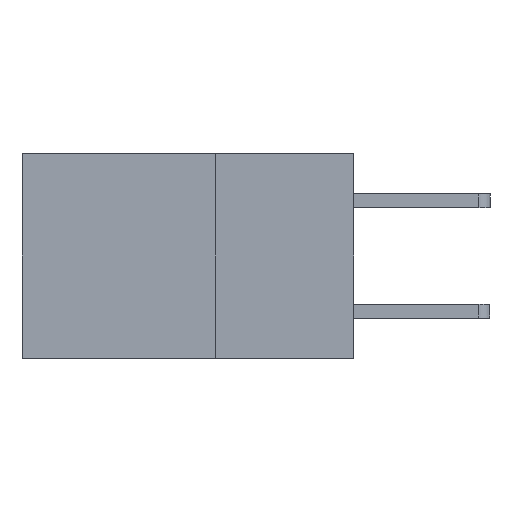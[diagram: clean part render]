
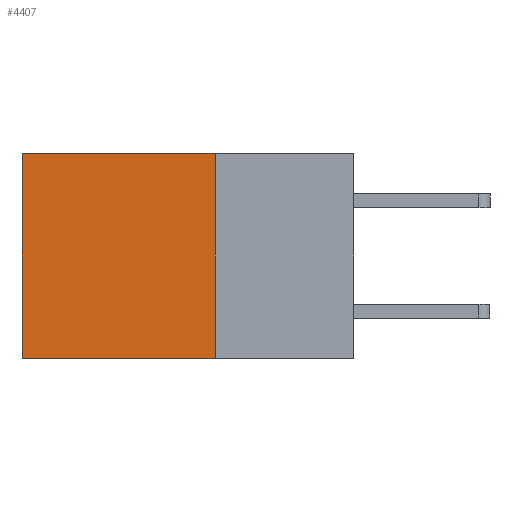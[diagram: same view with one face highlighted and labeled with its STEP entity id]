
A CAD part, left-side view. The second image highlights one B-rep face of the part: STEP entity #4407.
In plain terms, the highlighted planar face has unit normal (-1, 0, 0).
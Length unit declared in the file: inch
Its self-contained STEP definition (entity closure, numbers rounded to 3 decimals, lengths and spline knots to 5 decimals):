
#549 = DIRECTION ( 'NONE',  ( 0., 0., -1. ) ) ;
#629 = VECTOR ( 'NONE', #7844, 39.37008 ) ;
#669 = EDGE_CURVE ( 'NONE', #9523, #5300, #7351, .T. ) ;
#700 = CARTESIAN_POINT ( 'NONE',  ( 0.2875, 0.25, 0. ) ) ;
#918 = FACE_OUTER_BOUND ( 'NONE', #4464, .T. ) ;
#981 = VECTOR ( 'NONE', #4279, 39.37008 ) ;
#1225 = VERTEX_POINT ( 'NONE', #5848 ) ;
#1298 = DIRECTION ( 'NONE',  ( 0., 0., -1. ) ) ;
#1681 = DIRECTION ( 'NONE',  ( 1., 0., 0. ) ) ;
#2888 = CARTESIAN_POINT ( 'NONE',  ( 0.2875, 0.6, 0. ) ) ;
#3102 = ORIENTED_EDGE ( 'NONE', *, *, #7661, .T. ) ;
#3597 = LINE ( 'NONE', #2888, #9212 ) ;
#3654 = LINE ( 'NONE', #4520, #629 ) ;
#4135 = PLANE ( 'NONE',  #6755 ) ;
#4279 = DIRECTION ( 'NONE',  ( 0., 1., 0. ) ) ;
#4348 = CARTESIAN_POINT ( 'NONE',  ( 0.2875, 0.25, 0. ) ) ;
#4407 = ADVANCED_FACE ( 'NONE', ( #918 ), #4135, .F. ) ;
#4464 = EDGE_LOOP ( 'NONE', ( #3102, #5310, #4891, #7403 ) ) ;
#4520 = CARTESIAN_POINT ( 'NONE',  ( 0.2875, 0.25, -0.37 ) ) ;
#4877 = CARTESIAN_POINT ( 'NONE',  ( 0.2875, 0.6, -0.37 ) ) ;
#4891 = ORIENTED_EDGE ( 'NONE', *, *, #669, .F. ) ;
#5009 = DIRECTION ( 'NONE',  ( 0., 0., -1. ) ) ;
#5300 = VERTEX_POINT ( 'NONE', #7774 ) ;
#5310 = ORIENTED_EDGE ( 'NONE', *, *, #6019, .F. ) ;
#5842 = CARTESIAN_POINT ( 'NONE',  ( 0.2875, 0.25, 0. ) ) ;
#5848 = CARTESIAN_POINT ( 'NONE',  ( 0.2875, 0.6, 0. ) ) ;
#5897 = EDGE_CURVE ( 'NONE', #9523, #1225, #7730, .T. ) ;
#6019 = EDGE_CURVE ( 'NONE', #5300, #8237, #3654, .T. ) ;
#6755 = AXIS2_PLACEMENT_3D ( 'NONE', #4348, #1681, #5009 ) ;
#7351 = LINE ( 'NONE', #700, #7889 ) ;
#7403 = ORIENTED_EDGE ( 'NONE', *, *, #5897, .T. ) ;
#7661 = EDGE_CURVE ( 'NONE', #1225, #8237, #3597, .T. ) ;
#7730 = LINE ( 'NONE', #10072, #981 ) ;
#7774 = CARTESIAN_POINT ( 'NONE',  ( 0.2875, 0.25, -0.37 ) ) ;
#7844 = DIRECTION ( 'NONE',  ( 0., 1., 0. ) ) ;
#7889 = VECTOR ( 'NONE', #549, 39.37008 ) ;
#8237 = VERTEX_POINT ( 'NONE', #4877 ) ;
#9212 = VECTOR ( 'NONE', #1298, 39.37008 ) ;
#9523 = VERTEX_POINT ( 'NONE', #5842 ) ;
#10072 = CARTESIAN_POINT ( 'NONE',  ( 0.2875, 0.25, 0. ) ) ;
